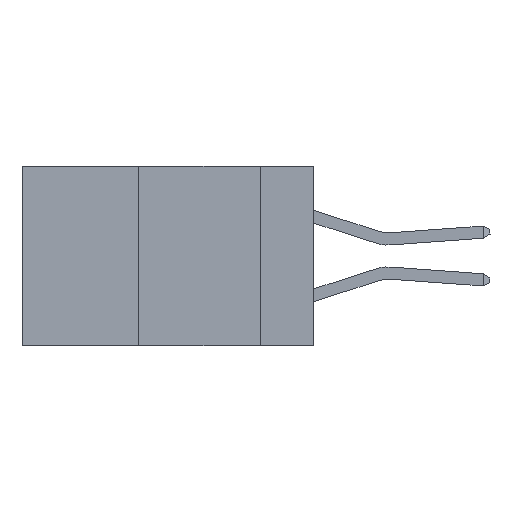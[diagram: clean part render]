
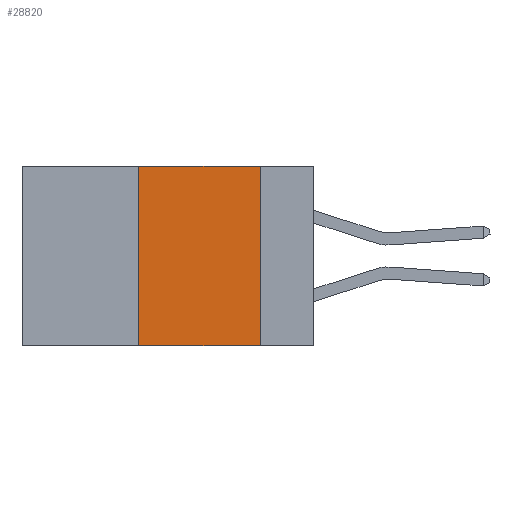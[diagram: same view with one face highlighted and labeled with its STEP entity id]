
A CAD part, left-side view. The second image highlights one B-rep face of the part: STEP entity #28820.
In plain terms, the highlighted planar face has unit normal (-1, 0, 0).
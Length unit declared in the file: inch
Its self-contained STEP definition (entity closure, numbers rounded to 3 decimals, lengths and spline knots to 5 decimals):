
#3737 = ORIENTED_EDGE ( 'NONE', *, *, #20128, .F. ) ;
#4036 = PLANE ( 'NONE',  #12164 ) ;
#7595 = DIRECTION ( 'NONE',  ( 0., 0., -1. ) ) ;
#8356 = DIRECTION ( 'NONE',  ( 0., 0., 1. ) ) ;
#8427 = VERTEX_POINT ( 'NONE', #14377 ) ;
#8955 = LINE ( 'NONE', #13383, #26850 ) ;
#10173 = EDGE_CURVE ( 'NONE', #8427, #29676, #8955, .T. ) ;
#10498 = LINE ( 'NONE', #28660, #28378 ) ;
#10589 = CARTESIAN_POINT ( 'NONE',  ( 0., 0.11, 0. ) ) ;
#10900 = VECTOR ( 'NONE', #8356, 39.37008 ) ;
#11152 = CARTESIAN_POINT ( 'NONE',  ( 0., 0.6, 0. ) ) ;
#11262 = DIRECTION ( 'NONE',  ( 0., 0., -1. ) ) ;
#11818 = LINE ( 'NONE', #19417, #18762 ) ;
#12164 = AXIS2_PLACEMENT_3D ( 'NONE', #11152, #25206, #11262 ) ;
#12319 = EDGE_CURVE ( 'NONE', #24981, #13174, #11818, .T. ) ;
#12398 = DIRECTION ( 'NONE',  ( 0., -1., 0. ) ) ;
#13174 = VERTEX_POINT ( 'NONE', #29325 ) ;
#13383 = CARTESIAN_POINT ( 'NONE',  ( 0., 0.6, 0. ) ) ;
#14377 = CARTESIAN_POINT ( 'NONE',  ( 0., 0.36, 0. ) ) ;
#15621 = ORIENTED_EDGE ( 'NONE', *, *, #10173, .F. ) ;
#16395 = LINE ( 'NONE', #17822, #10900 ) ;
#16442 = CARTESIAN_POINT ( 'NONE',  ( 0., 0.36, -0.37 ) ) ;
#17822 = CARTESIAN_POINT ( 'NONE',  ( 0., 0.36, 0. ) ) ;
#18762 = VECTOR ( 'NONE', #12398, 39.37008 ) ;
#19417 = CARTESIAN_POINT ( 'NONE',  ( 0., 0.6, -0.37 ) ) ;
#20128 = EDGE_CURVE ( 'NONE', #24981, #8427, #16395, .T. ) ;
#21054 = ORIENTED_EDGE ( 'NONE', *, *, #22495, .F. ) ;
#22495 = EDGE_CURVE ( 'NONE', #29676, #13174, #10498, .T. ) ;
#22522 = ORIENTED_EDGE ( 'NONE', *, *, #12319, .T. ) ;
#24374 = EDGE_LOOP ( 'NONE', ( #21054, #15621, #3737, #22522 ) ) ;
#24981 = VERTEX_POINT ( 'NONE', #16442 ) ;
#25206 = DIRECTION ( 'NONE',  ( 1., 0., 0. ) ) ;
#26850 = VECTOR ( 'NONE', #27290, 39.37008 ) ;
#27290 = DIRECTION ( 'NONE',  ( 0., -1., 0. ) ) ;
#27870 = FACE_OUTER_BOUND ( 'NONE', #24374, .T. ) ;
#28378 = VECTOR ( 'NONE', #7595, 39.37008 ) ;
#28660 = CARTESIAN_POINT ( 'NONE',  ( 0., 0.11, 0. ) ) ;
#28820 = ADVANCED_FACE ( 'NONE', ( #27870 ), #4036, .F. ) ;
#29325 = CARTESIAN_POINT ( 'NONE',  ( 0., 0.11, -0.37 ) ) ;
#29676 = VERTEX_POINT ( 'NONE', #10589 ) ;
